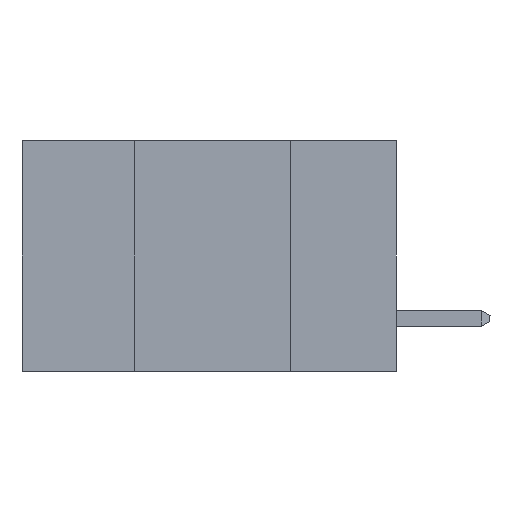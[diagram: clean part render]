
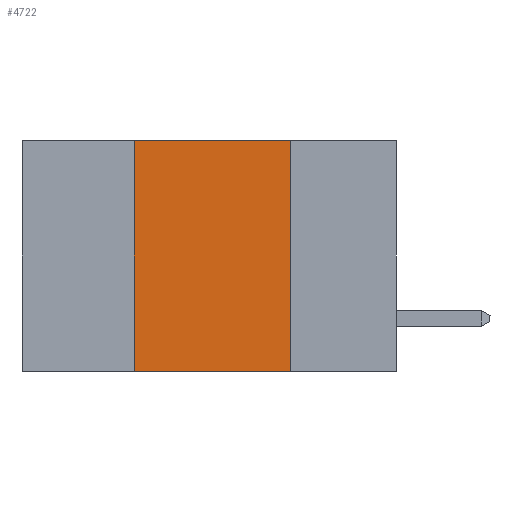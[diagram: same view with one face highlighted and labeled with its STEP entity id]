
A CAD part, left-side view. The second image highlights one B-rep face of the part: STEP entity #4722.
In plain terms, the highlighted planar face has unit normal (-1, 0, 0).
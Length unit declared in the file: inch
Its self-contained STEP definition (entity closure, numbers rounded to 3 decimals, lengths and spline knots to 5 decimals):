
#135 = ORIENTED_EDGE ( 'NONE', *, *, #9735, .T. ) ;
#995 = VERTEX_POINT ( 'NONE', #9537 ) ;
#2062 = CARTESIAN_POINT ( 'NONE',  ( 0., 0.17, -0.37 ) ) ;
#3493 = EDGE_LOOP ( 'NONE', ( #20823, #8016, #9361, #135 ) ) ;
#4030 = VECTOR ( 'NONE', #10769, 39.37008 ) ;
#4463 = CARTESIAN_POINT ( 'NONE',  ( 0., 0.6, 0. ) ) ;
#4566 = CARTESIAN_POINT ( 'NONE',  ( 0., 0.42, -0.37 ) ) ;
#4722 = ADVANCED_FACE ( 'NONE', ( #20713 ), #11879, .F. ) ;
#5314 = CARTESIAN_POINT ( 'NONE',  ( 0., 0.6, -0.37 ) ) ;
#5427 = EDGE_CURVE ( 'NONE', #6097, #14242, #14012, .T. ) ;
#6097 = VERTEX_POINT ( 'NONE', #10030 ) ;
#6690 = DIRECTION ( 'NONE',  ( 0., 0., 1. ) ) ;
#6702 = CARTESIAN_POINT ( 'NONE',  ( 0., 0.17, -0.37 ) ) ;
#8016 = ORIENTED_EDGE ( 'NONE', *, *, #16698, .F. ) ;
#9242 = VERTEX_POINT ( 'NONE', #4566 ) ;
#9361 = ORIENTED_EDGE ( 'NONE', *, *, #10076, .F. ) ;
#9383 = VECTOR ( 'NONE', #15254, 39.37008 ) ;
#9537 = CARTESIAN_POINT ( 'NONE',  ( 0., 0.42, 0. ) ) ;
#9735 = EDGE_CURVE ( 'NONE', #9242, #14242, #15877, .T. ) ;
#10030 = CARTESIAN_POINT ( 'NONE',  ( 0., 0.17, 0. ) ) ;
#10076 = EDGE_CURVE ( 'NONE', #9242, #995, #17250, .T. ) ;
#10769 = DIRECTION ( 'NONE',  ( 0., -1., 0. ) ) ;
#11665 = VECTOR ( 'NONE', #19496, 39.37008 ) ;
#11879 = PLANE ( 'NONE',  #17222 ) ;
#13401 = CARTESIAN_POINT ( 'NONE',  ( 0., 0.42, -0.37 ) ) ;
#13603 = DIRECTION ( 'NONE',  ( 0., 0., -1. ) ) ;
#14012 = LINE ( 'NONE', #2062, #11665 ) ;
#14242 = VERTEX_POINT ( 'NONE', #6702 ) ;
#15254 = DIRECTION ( 'NONE',  ( 0., -1., 0. ) ) ;
#15877 = LINE ( 'NONE', #5314, #4030 ) ;
#16698 = EDGE_CURVE ( 'NONE', #995, #6097, #18745, .T. ) ;
#16874 = DIRECTION ( 'NONE',  ( 1., 0., 0. ) ) ;
#17222 = AXIS2_PLACEMENT_3D ( 'NONE', #18743, #16874, #13603 ) ;
#17250 = LINE ( 'NONE', #13401, #19629 ) ;
#18743 = CARTESIAN_POINT ( 'NONE',  ( 0., 0.6, 0. ) ) ;
#18745 = LINE ( 'NONE', #4463, #9383 ) ;
#19496 = DIRECTION ( 'NONE',  ( 0., 0., -1. ) ) ;
#19629 = VECTOR ( 'NONE', #6690, 39.37008 ) ;
#20713 = FACE_OUTER_BOUND ( 'NONE', #3493, .T. ) ;
#20823 = ORIENTED_EDGE ( 'NONE', *, *, #5427, .F. ) ;
